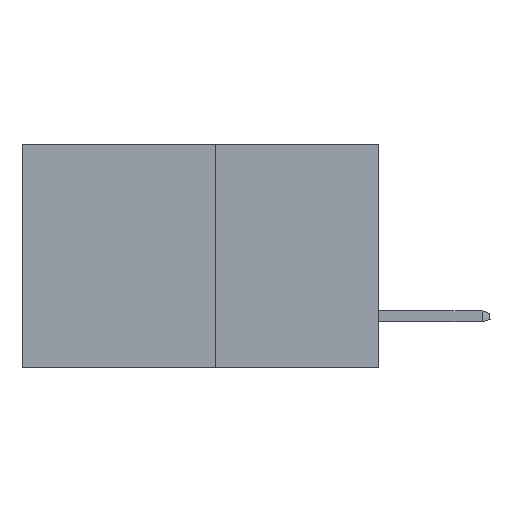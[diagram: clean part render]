
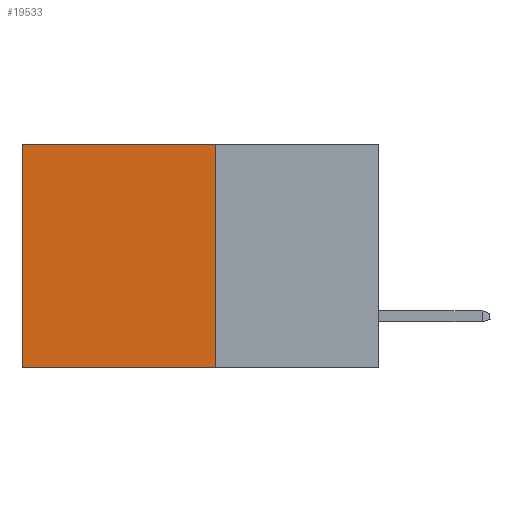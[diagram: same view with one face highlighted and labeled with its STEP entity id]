
A CAD part, left-side view. The second image highlights one B-rep face of the part: STEP entity #19533.
In plain terms, the highlighted planar face has unit normal (-1, 0, 0).
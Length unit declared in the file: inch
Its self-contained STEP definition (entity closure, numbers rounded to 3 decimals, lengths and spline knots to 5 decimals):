
#1548 = AXIS2_PLACEMENT_3D ( 'NONE', #10771, #4747, #15372 ) ;
#2637 = CARTESIAN_POINT ( 'NONE',  ( 0.277, 0.27, 0. ) ) ;
#2683 = VERTEX_POINT ( 'NONE', #3695 ) ;
#3503 = LINE ( 'NONE', #2637, #7494 ) ;
#3695 = CARTESIAN_POINT ( 'NONE',  ( 0.277, 0.27, -0.37 ) ) ;
#4280 = VECTOR ( 'NONE', #10718, 39.37008 ) ;
#4716 = VECTOR ( 'NONE', #5320, 39.37008 ) ;
#4747 = DIRECTION ( 'NONE',  ( 1., 0., 0. ) ) ;
#5184 = LINE ( 'NONE', #15954, #4716 ) ;
#5320 = DIRECTION ( 'NONE',  ( 0., 1., 0. ) ) ;
#5823 = EDGE_CURVE ( 'NONE', #15758, #2683, #8729, .T. ) ;
#6677 = EDGE_CURVE ( 'NONE', #2683, #9983, #5184, .T. ) ;
#7494 = VECTOR ( 'NONE', #13274, 39.37008 ) ;
#7685 = PLANE ( 'NONE',  #1548 ) ;
#8461 = CARTESIAN_POINT ( 'NONE',  ( 0.277, 0.27, -0.37 ) ) ;
#8608 = ORIENTED_EDGE ( 'NONE', *, *, #19348, .T. ) ;
#8729 = LINE ( 'NONE', #8461, #4280 ) ;
#8803 = CARTESIAN_POINT ( 'NONE',  ( 0.277, 0.59, -0.37 ) ) ;
#9983 = VERTEX_POINT ( 'NONE', #11657 ) ;
#10718 = DIRECTION ( 'NONE',  ( 0., 0., -1. ) ) ;
#10771 = CARTESIAN_POINT ( 'NONE',  ( 0.277, 0.27, -0.37 ) ) ;
#11424 = ORIENTED_EDGE ( 'NONE', *, *, #6677, .F. ) ;
#11568 = VERTEX_POINT ( 'NONE', #16172 ) ;
#11657 = CARTESIAN_POINT ( 'NONE',  ( 0.277, 0.59, -0.37 ) ) ;
#11960 = LINE ( 'NONE', #8803, #15995 ) ;
#13274 = DIRECTION ( 'NONE',  ( 0., 1., 0. ) ) ;
#13789 = ORIENTED_EDGE ( 'NONE', *, *, #14473, .T. ) ;
#14473 = EDGE_CURVE ( 'NONE', #15758, #11568, #3503, .T. ) ;
#15372 = DIRECTION ( 'NONE',  ( 0., 0., -1. ) ) ;
#15434 = ORIENTED_EDGE ( 'NONE', *, *, #5823, .F. ) ;
#15758 = VERTEX_POINT ( 'NONE', #16195 ) ;
#15954 = CARTESIAN_POINT ( 'NONE',  ( 0.277, 0.27, -0.37 ) ) ;
#15995 = VECTOR ( 'NONE', #19294, 39.37008 ) ;
#16172 = CARTESIAN_POINT ( 'NONE',  ( 0.277, 0.59, 0. ) ) ;
#16195 = CARTESIAN_POINT ( 'NONE',  ( 0.277, 0.27, 0. ) ) ;
#16208 = FACE_OUTER_BOUND ( 'NONE', #19383, .T. ) ;
#19294 = DIRECTION ( 'NONE',  ( 0., 0., -1. ) ) ;
#19348 = EDGE_CURVE ( 'NONE', #11568, #9983, #11960, .T. ) ;
#19383 = EDGE_LOOP ( 'NONE', ( #8608, #11424, #15434, #13789 ) ) ;
#19533 = ADVANCED_FACE ( 'NONE', ( #16208 ), #7685, .F. ) ;
